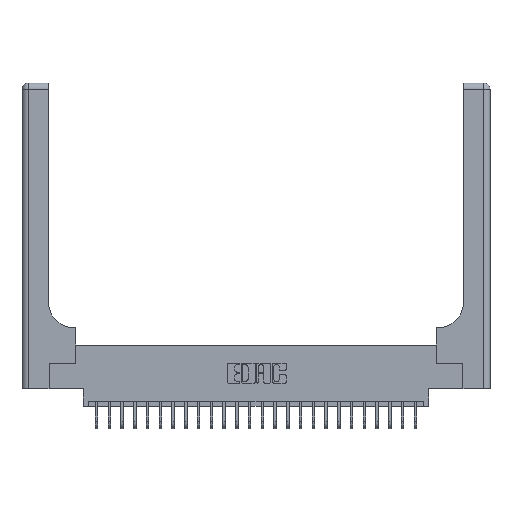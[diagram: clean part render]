
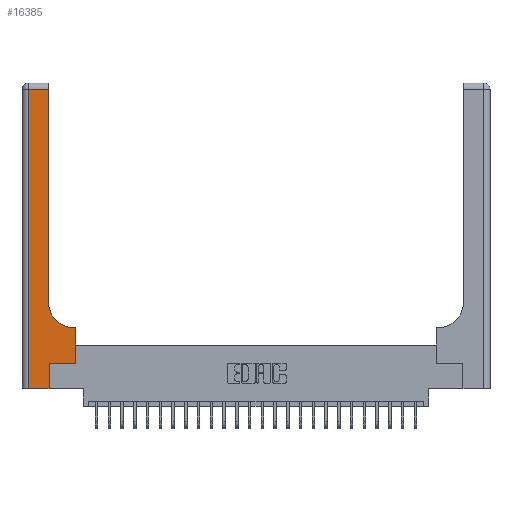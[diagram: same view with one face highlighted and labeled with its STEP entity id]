
A CAD part, top view. The second image highlights one B-rep face of the part: STEP entity #16385.
In plain terms, the highlighted planar face has unit normal (0, 0, 1).
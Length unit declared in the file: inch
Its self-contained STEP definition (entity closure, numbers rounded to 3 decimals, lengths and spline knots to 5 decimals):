
#360 = ORIENTED_EDGE ( 'NONE', *, *, #14227, .T. ) ;
#688 = VERTEX_POINT ( 'NONE', #5663 ) ;
#910 = VERTEX_POINT ( 'NONE', #20855 ) ;
#1364 = VECTOR ( 'NONE', #20216, 39.37008 ) ;
#1814 = VERTEX_POINT ( 'NONE', #12367 ) ;
#1941 = LINE ( 'NONE', #14614, #16937 ) ;
#2690 = VERTEX_POINT ( 'NONE', #14530 ) ;
#2887 = VERTEX_POINT ( 'NONE', #24215 ) ;
#2933 = ORIENTED_EDGE ( 'NONE', *, *, #25778, .T. ) ;
#3473 = ORIENTED_EDGE ( 'NONE', *, *, #20108, .T. ) ;
#3630 = DIRECTION ( 'NONE',  ( -1., 0., 0. ) ) ;
#3696 = AXIS2_PLACEMENT_3D ( 'NONE', #14170, #15990, #7693 ) ;
#3779 = DIRECTION ( 'NONE',  ( 1., 0., 0. ) ) ;
#4570 = VERTEX_POINT ( 'NONE', #19227 ) ;
#4572 = DIRECTION ( 'NONE',  ( -1., 0., 0. ) ) ;
#4640 = EDGE_CURVE ( 'NONE', #13111, #2690, #6276, .T. ) ;
#4890 = LINE ( 'NONE', #14253, #1364 ) ;
#5019 = CARTESIAN_POINT ( 'NONE',  ( 0.51, 0.6, 0.37 ) ) ;
#5290 = ORIENTED_EDGE ( 'NONE', *, *, #13358, .T. ) ;
#5659 = FACE_OUTER_BOUND ( 'NONE', #22719, .T. ) ;
#5663 = CARTESIAN_POINT ( 'NONE',  ( 0.26, 2.94, 0.37 ) ) ;
#6193 = DIRECTION ( 'NONE',  ( 0., 1., 0. ) ) ;
#6276 = CIRCLE ( 'NONE', #3696, 0.25 ) ;
#6412 = CARTESIAN_POINT ( 'NONE',  ( 0.26, 0.6, 0.37 ) ) ;
#6426 = VECTOR ( 'NONE', #13500, 39.37008 ) ;
#6822 = EDGE_CURVE ( 'NONE', #1814, #22662, #23934, .T. ) ;
#6917 = LINE ( 'NONE', #6412, #10455 ) ;
#7693 = DIRECTION ( 'NONE',  ( 1., 0., 0. ) ) ;
#8511 = CARTESIAN_POINT ( 'NONE',  ( 0.528, 0.25, 0.37 ) ) ;
#9794 = ORIENTED_EDGE ( 'NONE', *, *, #12837, .T. ) ;
#9800 = VECTOR ( 'NONE', #3779, 39.37008 ) ;
#9833 = EDGE_CURVE ( 'NONE', #22662, #4570, #13968, .T. ) ;
#10455 = VECTOR ( 'NONE', #4572, 39.37008 ) ;
#11375 = DIRECTION ( 'NONE',  ( -1., 0., 0. ) ) ;
#11464 = LINE ( 'NONE', #18402, #21591 ) ;
#11517 = LINE ( 'NONE', #13272, #19751 ) ;
#12367 = CARTESIAN_POINT ( 'NONE',  ( 0.06, 2.94, 0.37 ) ) ;
#12837 = EDGE_CURVE ( 'NONE', #2887, #19441, #4890, .T. ) ;
#13111 = VERTEX_POINT ( 'NONE', #5019 ) ;
#13174 = LINE ( 'NONE', #17805, #6426 ) ;
#13272 = CARTESIAN_POINT ( 'NONE',  ( 0., 2.94, 0.37 ) ) ;
#13358 = EDGE_CURVE ( 'NONE', #4570, #2887, #13174, .T. ) ;
#13500 = DIRECTION ( 'NONE',  ( 0., 1., 0. ) ) ;
#13968 = LINE ( 'NONE', #15956, #9800 ) ;
#14170 = CARTESIAN_POINT ( 'NONE',  ( 0.51, 0.85, 0.37 ) ) ;
#14227 = EDGE_CURVE ( 'NONE', #19441, #910, #1941, .T. ) ;
#14235 = DIRECTION ( 'NONE',  ( 0., -1., 0. ) ) ;
#14253 = CARTESIAN_POINT ( 'NONE',  ( 0.265, 0.25, 0.37 ) ) ;
#14530 = CARTESIAN_POINT ( 'NONE',  ( 0.26, 0.85, 0.37 ) ) ;
#14614 = CARTESIAN_POINT ( 'NONE',  ( 0.528, 0.25, 0.37 ) ) ;
#14705 = DIRECTION ( 'NONE',  ( 0., 1., 0. ) ) ;
#15218 = EDGE_CURVE ( 'NONE', #2690, #688, #11464, .T. ) ;
#15956 = CARTESIAN_POINT ( 'NONE',  ( 0., 0., 0.37 ) ) ;
#15990 = DIRECTION ( 'NONE',  ( 0., 0., -1. ) ) ;
#16385 = ADVANCED_FACE ( 'NONE', ( #5659 ), #19358, .F. ) ;
#16937 = VECTOR ( 'NONE', #14705, 39.37008 ) ;
#17425 = DIRECTION ( 'NONE',  ( 0., 0., -1. ) ) ;
#17805 = CARTESIAN_POINT ( 'NONE',  ( 0.265, 0., 0.37 ) ) ;
#18402 = CARTESIAN_POINT ( 'NONE',  ( 0.26, 3., 0.37 ) ) ;
#19227 = CARTESIAN_POINT ( 'NONE',  ( 0.265, 0., 0.37 ) ) ;
#19358 = PLANE ( 'NONE',  #20993 ) ;
#19441 = VERTEX_POINT ( 'NONE', #8511 ) ;
#19514 = ORIENTED_EDGE ( 'NONE', *, *, #4640, .T. ) ;
#19751 = VECTOR ( 'NONE', #3630, 39.37008 ) ;
#20108 = EDGE_CURVE ( 'NONE', #910, #13111, #6917, .T. ) ;
#20216 = DIRECTION ( 'NONE',  ( 1., 0., 0. ) ) ;
#20855 = CARTESIAN_POINT ( 'NONE',  ( 0.528, 0.6, 0.37 ) ) ;
#20993 = AXIS2_PLACEMENT_3D ( 'NONE', #23312, #17425, #11375 ) ;
#21591 = VECTOR ( 'NONE', #6193, 39.37008 ) ;
#21651 = ORIENTED_EDGE ( 'NONE', *, *, #9833, .T. ) ;
#22226 = CARTESIAN_POINT ( 'NONE',  ( 0.06, 3., 0.37 ) ) ;
#22662 = VERTEX_POINT ( 'NONE', #23961 ) ;
#22719 = EDGE_LOOP ( 'NONE', ( #23516, #2933, #25377, #21651, #5290, #9794, #360, #3473, #19514 ) ) ;
#23312 = CARTESIAN_POINT ( 'NONE',  ( 0., 3., 0.37 ) ) ;
#23516 = ORIENTED_EDGE ( 'NONE', *, *, #15218, .T. ) ;
#23934 = LINE ( 'NONE', #22226, #25808 ) ;
#23961 = CARTESIAN_POINT ( 'NONE',  ( 0.06, 0., 0.37 ) ) ;
#24215 = CARTESIAN_POINT ( 'NONE',  ( 0.265, 0.25, 0.37 ) ) ;
#25377 = ORIENTED_EDGE ( 'NONE', *, *, #6822, .T. ) ;
#25778 = EDGE_CURVE ( 'NONE', #688, #1814, #11517, .T. ) ;
#25808 = VECTOR ( 'NONE', #14235, 39.37008 ) ;
